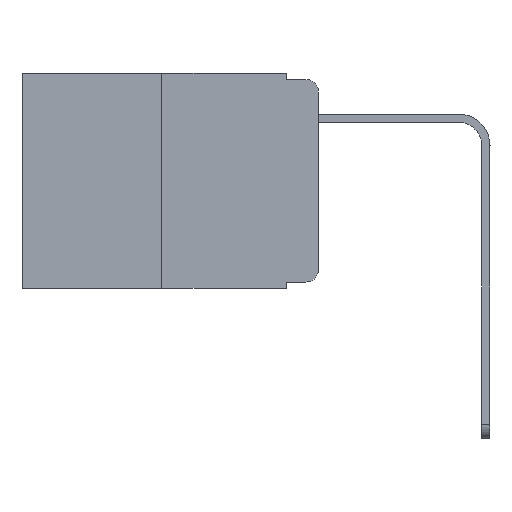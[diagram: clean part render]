
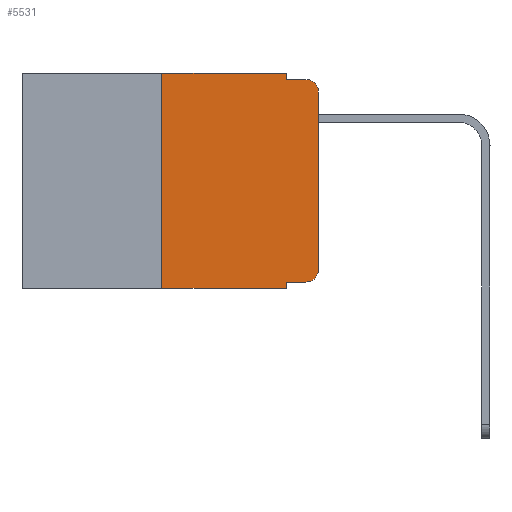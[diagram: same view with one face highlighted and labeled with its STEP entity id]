
A CAD part, left-side view. The second image highlights one B-rep face of the part: STEP entity #5531.
In plain terms, the highlighted planar face has unit normal (-1, 0, 0).
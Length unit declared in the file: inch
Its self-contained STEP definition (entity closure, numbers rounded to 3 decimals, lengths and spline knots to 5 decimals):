
#132 = LINE ( 'NONE', #13692, #8633 ) ;
#202 = EDGE_CURVE ( 'NONE', #20212, #9455, #1268, .T. ) ;
#395 = LINE ( 'NONE', #17762, #3827 ) ;
#478 = CARTESIAN_POINT ( 'NONE',  ( 0., 0.25, -0.343 ) ) ;
#609 = ORIENTED_EDGE ( 'NONE', *, *, #6134, .T. ) ;
#911 = CARTESIAN_POINT ( 'NONE',  ( 0., 0.051, -0.01 ) ) ;
#1044 = ORIENTED_EDGE ( 'NONE', *, *, #202, .T. ) ;
#1268 = LINE ( 'NONE', #9358, #13302 ) ;
#1457 = CARTESIAN_POINT ( 'NONE',  ( 0., 0., 0. ) ) ;
#1669 = CARTESIAN_POINT ( 'NONE',  ( 0., 0.02, -0.333 ) ) ;
#1935 = EDGE_CURVE ( 'NONE', #20212, #6750, #132, .T. ) ;
#2144 = CARTESIAN_POINT ( 'NONE',  ( 0., 0.02, -0.01 ) ) ;
#2186 = DIRECTION ( 'NONE',  ( 1., 0., 0. ) ) ;
#2426 = DIRECTION ( 'NONE',  ( 0., 0., -1. ) ) ;
#2441 = ORIENTED_EDGE ( 'NONE', *, *, #12365, .T. ) ;
#2633 = CIRCLE ( 'NONE', #3781, 0.02 ) ;
#2692 = LINE ( 'NONE', #1457, #6693 ) ;
#2894 = ORIENTED_EDGE ( 'NONE', *, *, #20311, .F. ) ;
#3337 = CARTESIAN_POINT ( 'NONE',  ( 0., 0.051, 0. ) ) ;
#3389 = DIRECTION ( 'NONE',  ( 0., -1., 0. ) ) ;
#3393 = EDGE_CURVE ( 'NONE', #7011, #18560, #2692, .T. ) ;
#3496 = DIRECTION ( 'NONE',  ( 0., 0., -1. ) ) ;
#3781 = AXIS2_PLACEMENT_3D ( 'NONE', #13528, #15453, #8584 ) ;
#3827 = VECTOR ( 'NONE', #9405, 39.37008 ) ;
#4078 = CARTESIAN_POINT ( 'NONE',  ( 0., 0.02, -0.03 ) ) ;
#4554 = AXIS2_PLACEMENT_3D ( 'NONE', #10789, #2186, #10643 ) ;
#4720 = LINE ( 'NONE', #3337, #9027 ) ;
#4764 = CARTESIAN_POINT ( 'NONE',  ( 0., 0.051, 0. ) ) ;
#5440 = ORIENTED_EDGE ( 'NONE', *, *, #3393, .T. ) ;
#5531 = ADVANCED_FACE ( 'NONE', ( #18999 ), #10718, .F. ) ;
#6134 = EDGE_CURVE ( 'NONE', #18560, #16196, #20283, .T. ) ;
#6665 = CARTESIAN_POINT ( 'NONE',  ( 0., 0.473, 0. ) ) ;
#6693 = VECTOR ( 'NONE', #9842, 39.37008 ) ;
#6709 = VECTOR ( 'NONE', #7012, 39.37008 ) ;
#6750 = VERTEX_POINT ( 'NONE', #12371 ) ;
#7011 = VERTEX_POINT ( 'NONE', #18365 ) ;
#7012 = DIRECTION ( 'NONE',  ( 0., 0., -1. ) ) ;
#7316 = LINE ( 'NONE', #6665, #14315 ) ;
#7571 = DIRECTION ( 'NONE',  ( -1., 0., 0. ) ) ;
#7768 = CARTESIAN_POINT ( 'NONE',  ( 0., 0.051, -0.333 ) ) ;
#7837 = EDGE_CURVE ( 'NONE', #6750, #10076, #7316, .T. ) ;
#8305 = ORIENTED_EDGE ( 'NONE', *, *, #1935, .F. ) ;
#8584 = DIRECTION ( 'NONE',  ( 0., 0., -1. ) ) ;
#8612 = DIRECTION ( 'NONE',  ( 0., -1., 0. ) ) ;
#8633 = VECTOR ( 'NONE', #13997, 39.37008 ) ;
#9027 = VECTOR ( 'NONE', #3496, 39.37008 ) ;
#9358 = CARTESIAN_POINT ( 'NONE',  ( 0., 0.473, -0.343 ) ) ;
#9405 = DIRECTION ( 'NONE',  ( 0., -1., 0. ) ) ;
#9455 = VERTEX_POINT ( 'NONE', #11468 ) ;
#9559 = CARTESIAN_POINT ( 'NONE',  ( 0., 0.051, -0.01 ) ) ;
#9842 = DIRECTION ( 'NONE',  ( 0., 0., 1. ) ) ;
#10076 = VERTEX_POINT ( 'NONE', #4764 ) ;
#10216 = EDGE_CURVE ( 'NONE', #18020, #7011, #2633, .T. ) ;
#10643 = DIRECTION ( 'NONE',  ( 0., 0., -1. ) ) ;
#10644 = VERTEX_POINT ( 'NONE', #9559 ) ;
#10718 = PLANE ( 'NONE',  #4554 ) ;
#10752 = ORIENTED_EDGE ( 'NONE', *, *, #13253, .F. ) ;
#10789 = CARTESIAN_POINT ( 'NONE',  ( 0., 0.473, 0. ) ) ;
#11468 = CARTESIAN_POINT ( 'NONE',  ( 0., 0.051, -0.343 ) ) ;
#12365 = EDGE_CURVE ( 'NONE', #19786, #18020, #395, .T. ) ;
#12371 = CARTESIAN_POINT ( 'NONE',  ( 0., 0.25, 0. ) ) ;
#13253 = EDGE_CURVE ( 'NONE', #10076, #10644, #19112, .T. ) ;
#13302 = VECTOR ( 'NONE', #8612, 39.37008 ) ;
#13496 = VECTOR ( 'NONE', #19790, 39.37008 ) ;
#13528 = CARTESIAN_POINT ( 'NONE',  ( 0., 0.02, -0.313 ) ) ;
#13692 = CARTESIAN_POINT ( 'NONE',  ( 0., 0.25, 0. ) ) ;
#13997 = DIRECTION ( 'NONE',  ( 0., 0., 1. ) ) ;
#14315 = VECTOR ( 'NONE', #3389, 39.37008 ) ;
#14330 = EDGE_LOOP ( 'NONE', ( #5440, #609, #2894, #10752, #18479, #8305, #1044, #15037, #2441, #18927 ) ) ;
#15037 = ORIENTED_EDGE ( 'NONE', *, *, #18667, .F. ) ;
#15453 = DIRECTION ( 'NONE',  ( -1., 0., 0. ) ) ;
#16196 = VERTEX_POINT ( 'NONE', #2144 ) ;
#16784 = CARTESIAN_POINT ( 'NONE',  ( 0., 0., -0.03 ) ) ;
#17762 = CARTESIAN_POINT ( 'NONE',  ( 0., 0.051, -0.333 ) ) ;
#18020 = VERTEX_POINT ( 'NONE', #1669 ) ;
#18107 = LINE ( 'NONE', #911, #13496 ) ;
#18365 = CARTESIAN_POINT ( 'NONE',  ( 0., 0., -0.313 ) ) ;
#18479 = ORIENTED_EDGE ( 'NONE', *, *, #7837, .F. ) ;
#18560 = VERTEX_POINT ( 'NONE', #16784 ) ;
#18611 = CARTESIAN_POINT ( 'NONE',  ( 0., 0.051, 0. ) ) ;
#18667 = EDGE_CURVE ( 'NONE', #19786, #9455, #4720, .T. ) ;
#18927 = ORIENTED_EDGE ( 'NONE', *, *, #10216, .T. ) ;
#18999 = FACE_OUTER_BOUND ( 'NONE', #14330, .T. ) ;
#19112 = LINE ( 'NONE', #18611, #6709 ) ;
#19786 = VERTEX_POINT ( 'NONE', #7768 ) ;
#19790 = DIRECTION ( 'NONE',  ( 0., -1., 0. ) ) ;
#20212 = VERTEX_POINT ( 'NONE', #478 ) ;
#20283 = CIRCLE ( 'NONE', #21681, 0.02 ) ;
#20311 = EDGE_CURVE ( 'NONE', #10644, #16196, #18107, .T. ) ;
#21681 = AXIS2_PLACEMENT_3D ( 'NONE', #4078, #7571, #2426 ) ;
